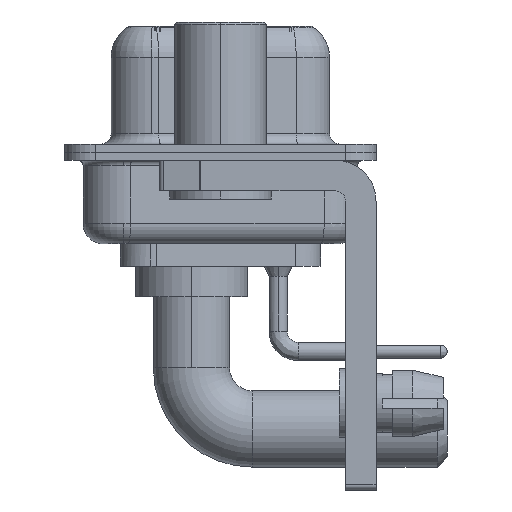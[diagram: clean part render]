
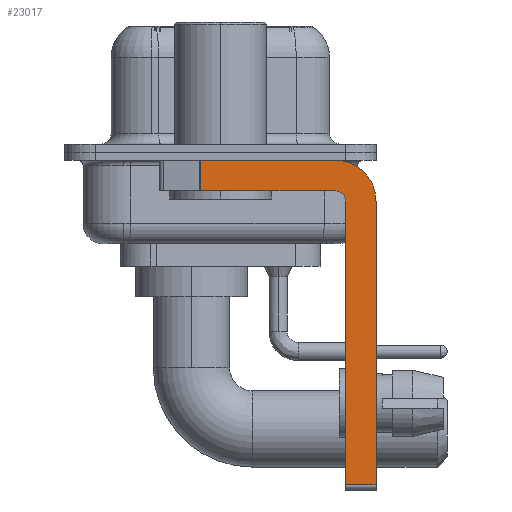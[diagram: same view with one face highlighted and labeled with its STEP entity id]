
A CAD part, left-side view. The second image highlights one B-rep face of the part: STEP entity #23017.
In plain terms, the highlighted planar face has unit normal (-1, 0, 0).
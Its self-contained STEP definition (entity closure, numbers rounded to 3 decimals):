
#829 = VECTOR ( 'NONE', #2294, 1000. ) ;
#2294 = DIRECTION ( 'NONE',  ( 0., 0., -1. ) ) ;
#2671 = EDGE_LOOP ( 'NONE', ( #15701, #15829, #18832, #6128, #15824, #21623, #19147, #18053 ) ) ;
#2941 = PLANE ( 'NONE',  #6549 ) ;
#3337 = VERTEX_POINT ( 'NONE', #6211 ) ;
#3444 = CARTESIAN_POINT ( 'NONE',  ( -2.9, -5.65, -1.9 ) ) ;
#3585 = CARTESIAN_POINT ( 'NONE',  ( -2.9, 3., -0.4 ) ) ;
#3696 = VERTEX_POINT ( 'NONE', #24227 ) ;
#4441 = DIRECTION ( 'NONE',  ( 0., 0., -1. ) ) ;
#4878 = CARTESIAN_POINT ( 'NONE',  ( -2.9, -5.65, -2.4 ) ) ;
#5444 = EDGE_CURVE ( 'NONE', #3696, #14898, #14242, .T. ) ;
#5640 = AXIS2_PLACEMENT_3D ( 'NONE', #17094, #17220, #15162 ) ;
#5858 = DIRECTION ( 'NONE',  ( 0., 0., 1. ) ) ;
#6127 = EDGE_CURVE ( 'NONE', #3337, #13171, #23063, .T. ) ;
#6128 = ORIENTED_EDGE ( 'NONE', *, *, #19053, .F. ) ;
#6211 = CARTESIAN_POINT ( 'NONE',  ( -2.9, -5.65, -1.9 ) ) ;
#6549 = AXIS2_PLACEMENT_3D ( 'NONE', #4878, #22317, #12221 ) ;
#7533 = CARTESIAN_POINT ( 'NONE',  ( -2.9, -7.65, -16.35 ) ) ;
#8314 = DIRECTION ( 'NONE',  ( 0., 0., 1. ) ) ;
#9231 = CARTESIAN_POINT ( 'NONE',  ( -2.9, -7.65, -2.4 ) ) ;
#9361 = DIRECTION ( 'NONE',  ( 0., 1., 0. ) ) ;
#9721 = DIRECTION ( 'NONE',  ( -1., 0., 0. ) ) ;
#11389 = CARTESIAN_POINT ( 'NONE',  ( -2.9, -5.65, -2.4 ) ) ;
#12221 = DIRECTION ( 'NONE',  ( 0., 0., -1. ) ) ;
#12611 = CARTESIAN_POINT ( 'NONE',  ( -2.9, 0.978, -1.9 ) ) ;
#12744 = VECTOR ( 'NONE', #4441, 1000. ) ;
#12831 = VERTEX_POINT ( 'NONE', #20950 ) ;
#13046 = VECTOR ( 'NONE', #9361, 1000. ) ;
#13171 = VERTEX_POINT ( 'NONE', #12611 ) ;
#13864 = LINE ( 'NONE', #21675, #829 ) ;
#14242 = CIRCLE ( 'NONE', #5640, 2. ) ;
#14339 = CIRCLE ( 'NONE', #17197, 0.5 ) ;
#14846 = EDGE_CURVE ( 'NONE', #24131, #15238, #22971, .T. ) ;
#14881 = LINE ( 'NONE', #9231, #12744 ) ;
#14898 = VERTEX_POINT ( 'NONE', #16845 ) ;
#15010 = VECTOR ( 'NONE', #16970, 1000. ) ;
#15162 = DIRECTION ( 'NONE',  ( 0., 0., -1. ) ) ;
#15238 = VERTEX_POINT ( 'NONE', #7533 ) ;
#15701 = ORIENTED_EDGE ( 'NONE', *, *, #23167, .F. ) ;
#15824 = ORIENTED_EDGE ( 'NONE', *, *, #25000, .F. ) ;
#15829 = ORIENTED_EDGE ( 'NONE', *, *, #22554, .T. ) ;
#16541 = LINE ( 'NONE', #22414, #18539 ) ;
#16845 = CARTESIAN_POINT ( 'NONE',  ( -2.9, -7.65, -2.4 ) ) ;
#16970 = DIRECTION ( 'NONE',  ( 0., -1., 0. ) ) ;
#17094 = CARTESIAN_POINT ( 'NONE',  ( -2.9, -5.65, -2.4 ) ) ;
#17197 = AXIS2_PLACEMENT_3D ( 'NONE', #11389, #9721, #5858 ) ;
#17220 = DIRECTION ( 'NONE',  ( 1., 0., 0. ) ) ;
#17723 = VERTEX_POINT ( 'NONE', #22124 ) ;
#18053 = ORIENTED_EDGE ( 'NONE', *, *, #5444, .F. ) ;
#18539 = VECTOR ( 'NONE', #8314, 1000. ) ;
#18832 = ORIENTED_EDGE ( 'NONE', *, *, #6127, .F. ) ;
#19053 = EDGE_CURVE ( 'NONE', #12831, #3337, #14339, .T. ) ;
#19147 = ORIENTED_EDGE ( 'NONE', *, *, #23265, .F. ) ;
#20805 = CARTESIAN_POINT ( 'NONE',  ( -2.9, -5.65, -16.35 ) ) ;
#20950 = CARTESIAN_POINT ( 'NONE',  ( -2.9, -6.15, -2.4 ) ) ;
#21623 = ORIENTED_EDGE ( 'NONE', *, *, #14846, .T. ) ;
#21675 = CARTESIAN_POINT ( 'NONE',  ( -2.9, 0.978, -1.9 ) ) ;
#22124 = CARTESIAN_POINT ( 'NONE',  ( -2.9, 0.978, -0.4 ) ) ;
#22317 = DIRECTION ( 'NONE',  ( 1., 0., 0. ) ) ;
#22414 = CARTESIAN_POINT ( 'NONE',  ( -2.9, -6.15, -16.6 ) ) ;
#22554 = EDGE_CURVE ( 'NONE', #17723, #13171, #13864, .T. ) ;
#22971 = LINE ( 'NONE', #20805, #15010 ) ;
#23017 = ADVANCED_FACE ( 'NONE', ( #24115 ), #2941, .F. ) ;
#23063 = LINE ( 'NONE', #3444, #13046 ) ;
#23167 = EDGE_CURVE ( 'NONE', #17723, #3696, #24494, .T. ) ;
#23265 = EDGE_CURVE ( 'NONE', #14898, #15238, #14881, .T. ) ;
#23779 = VECTOR ( 'NONE', #24879, 1000. ) ;
#24115 = FACE_OUTER_BOUND ( 'NONE', #2671, .T. ) ;
#24131 = VERTEX_POINT ( 'NONE', #25041 ) ;
#24227 = CARTESIAN_POINT ( 'NONE',  ( -2.9, -5.65, -0.4 ) ) ;
#24494 = LINE ( 'NONE', #3585, #23779 ) ;
#24879 = DIRECTION ( 'NONE',  ( 0., -1., 0. ) ) ;
#25000 = EDGE_CURVE ( 'NONE', #24131, #12831, #16541, .T. ) ;
#25041 = CARTESIAN_POINT ( 'NONE',  ( -2.9, -6.15, -16.35 ) ) ;
